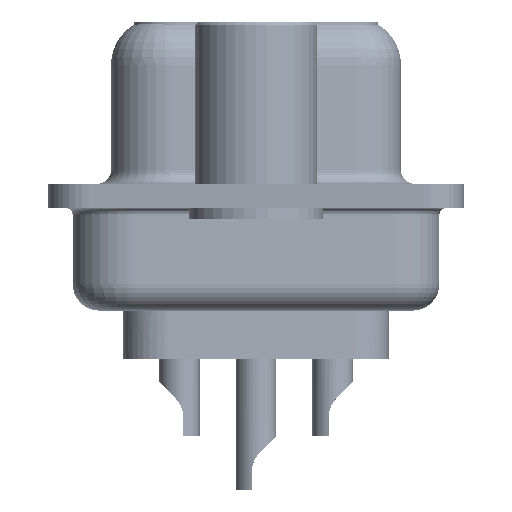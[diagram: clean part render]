
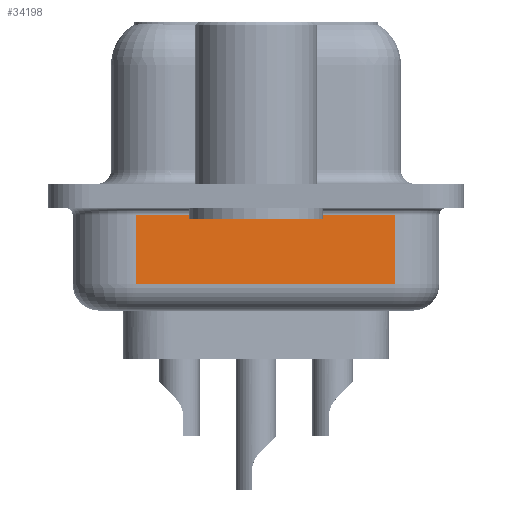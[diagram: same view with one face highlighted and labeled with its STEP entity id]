
A CAD part, left-side view. The second image highlights one B-rep face of the part: STEP entity #34198.
In plain terms, the highlighted planar face has unit normal (-0.985, -0.174, 0).
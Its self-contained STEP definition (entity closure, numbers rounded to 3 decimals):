
#318 = LINE ( 'NONE', #24969, #38265 ) ;
#937 = DIRECTION ( 'NONE',  ( 0., 0., 1. ) ) ;
#1035 = DIRECTION ( 'NONE',  ( -0.174, 0.985, 0. ) ) ;
#2951 = VERTEX_POINT ( 'NONE', #9447 ) ;
#3889 = VERTEX_POINT ( 'NONE', #30182 ) ;
#3976 = CARTESIAN_POINT ( 'NONE',  ( 2.93, 4.453, -0.7 ) ) ;
#4098 = DIRECTION ( 'NONE',  ( 0.174, -0.985, 0. ) ) ;
#4980 = ORIENTED_EDGE ( 'NONE', *, *, #28069, .T. ) ;
#7713 = CARTESIAN_POINT ( 'NONE',  ( 4.623, -5.147, -4.25 ) ) ;
#7902 = LINE ( 'NONE', #30933, #22921 ) ;
#9447 = CARTESIAN_POINT ( 'NONE',  ( 2.93, 4.453, -3.25 ) ) ;
#11997 = LINE ( 'NONE', #7713, #26949 ) ;
#13785 = VECTOR ( 'NONE', #17114, 1000. ) ;
#14850 = EDGE_CURVE ( 'NONE', #2951, #33514, #318, .T. ) ;
#16906 = ORIENTED_EDGE ( 'NONE', *, *, #14850, .F. ) ;
#17114 = DIRECTION ( 'NONE',  ( -0.174, 0.985, 0. ) ) ;
#19111 = DIRECTION ( 'NONE',  ( 0.985, 0.174, 0. ) ) ;
#21653 = EDGE_CURVE ( 'NONE', #3889, #33514, #21802, .T. ) ;
#21692 = CARTESIAN_POINT ( 'NONE',  ( 4.623, -5.147, -3.25 ) ) ;
#21802 = LINE ( 'NONE', #28919, #13785 ) ;
#22343 = ORIENTED_EDGE ( 'NONE', *, *, #21653, .T. ) ;
#22374 = EDGE_LOOP ( 'NONE', ( #16906, #22985, #4980, #22343 ) ) ;
#22661 = DIRECTION ( 'NONE',  ( 0., 0., 1. ) ) ;
#22921 = VECTOR ( 'NONE', #4098, 1000. ) ;
#22985 = ORIENTED_EDGE ( 'NONE', *, *, #33549, .T. ) ;
#24969 = CARTESIAN_POINT ( 'NONE',  ( 2.93, 4.453, -4.25 ) ) ;
#26949 = VECTOR ( 'NONE', #22661, 1000. ) ;
#27908 = PLANE ( 'NONE',  #38447 ) ;
#28069 = EDGE_CURVE ( 'NONE', #31262, #3889, #11997, .T. ) ;
#28919 = CARTESIAN_POINT ( 'NONE',  ( 2.93, 4.453, -0.7 ) ) ;
#30182 = CARTESIAN_POINT ( 'NONE',  ( 4.623, -5.147, -0.7 ) ) ;
#30933 = CARTESIAN_POINT ( 'NONE',  ( 2.93, 4.453, -3.25 ) ) ;
#31262 = VERTEX_POINT ( 'NONE', #21692 ) ;
#31677 = FACE_OUTER_BOUND ( 'NONE', #22374, .T. ) ;
#33514 = VERTEX_POINT ( 'NONE', #3976 ) ;
#33549 = EDGE_CURVE ( 'NONE', #2951, #31262, #7902, .T. ) ;
#34198 = ADVANCED_FACE ( 'NONE', ( #31677 ), #27908, .F. ) ;
#36924 = CARTESIAN_POINT ( 'NONE',  ( 2.93, 4.453, -4.25 ) ) ;
#38265 = VECTOR ( 'NONE', #937, 1000. ) ;
#38447 = AXIS2_PLACEMENT_3D ( 'NONE', #36924, #19111, #1035 ) ;
